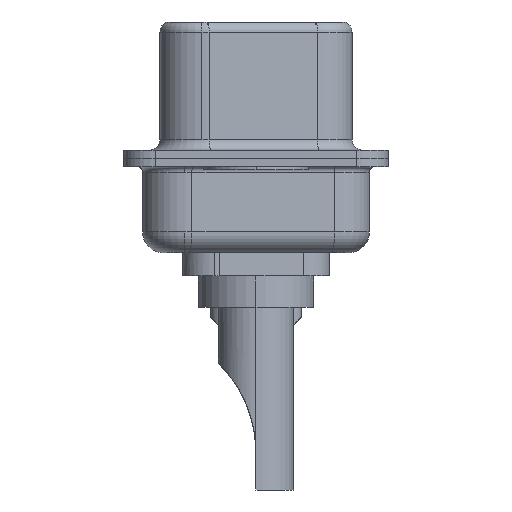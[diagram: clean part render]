
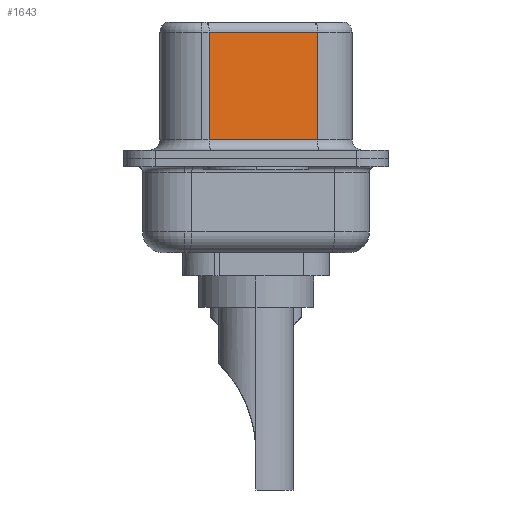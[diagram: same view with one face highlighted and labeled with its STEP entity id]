
A CAD part, left-side view. The second image highlights one B-rep face of the part: STEP entity #1643.
In plain terms, the highlighted planar face has unit normal (-0.985, -0.174, 0).
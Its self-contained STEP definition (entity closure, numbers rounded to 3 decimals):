
#1643 = ADVANCED_FACE ( 'NONE', ( #7416 ), #1813, .F. ) ;
#1660 = EDGE_CURVE ( 'NONE', #17910, #2416, #16244, .T. ) ;
#1813 = PLANE ( 'NONE',  #17124 ) ;
#1856 = CARTESIAN_POINT ( 'NONE',  ( 4.58, -2.927, 6.52 ) ) ;
#2416 = VERTEX_POINT ( 'NONE', #5409 ) ;
#3544 = CARTESIAN_POINT ( 'NONE',  ( 4.58, -2.927, 6.02 ) ) ;
#3776 = VERTEX_POINT ( 'NONE', #17228 ) ;
#3906 = DIRECTION ( 'NONE',  ( -0.174, 0.985, 0. ) ) ;
#4386 = EDGE_CURVE ( 'NONE', #17910, #3776, #13845, .T. ) ;
#4567 = CARTESIAN_POINT ( 'NONE',  ( 4.58, -2.927, 6.02 ) ) ;
#5299 = VECTOR ( 'NONE', #16974, 1000. ) ;
#5409 = CARTESIAN_POINT ( 'NONE',  ( 3.67, 2.233, 6.02 ) ) ;
#5668 = EDGE_CURVE ( 'NONE', #2416, #12429, #13538, .T. ) ;
#6382 = ORIENTED_EDGE ( 'NONE', *, *, #4386, .F. ) ;
#7416 = FACE_OUTER_BOUND ( 'NONE', #19890, .T. ) ;
#9119 = DIRECTION ( 'NONE',  ( 0., 0., -1. ) ) ;
#9835 = LINE ( 'NONE', #10320, #5299 ) ;
#10320 = CARTESIAN_POINT ( 'NONE',  ( 4.58, -2.927, 0.9 ) ) ;
#12429 = VERTEX_POINT ( 'NONE', #21660 ) ;
#13538 = LINE ( 'NONE', #16233, #21734 ) ;
#13790 = ORIENTED_EDGE ( 'NONE', *, *, #1660, .T. ) ;
#13845 = LINE ( 'NONE', #15542, #17678 ) ;
#14345 = ORIENTED_EDGE ( 'NONE', *, *, #5668, .T. ) ;
#15120 = ORIENTED_EDGE ( 'NONE', *, *, #19534, .T. ) ;
#15542 = CARTESIAN_POINT ( 'NONE',  ( 4.58, -2.927, 6.52 ) ) ;
#15750 = VECTOR ( 'NONE', #3906, 1000. ) ;
#16165 = DIRECTION ( 'NONE',  ( 0., 0., -1. ) ) ;
#16233 = CARTESIAN_POINT ( 'NONE',  ( 3.67, 2.233, 6.52 ) ) ;
#16244 = LINE ( 'NONE', #4567, #15750 ) ;
#16762 = DIRECTION ( 'NONE',  ( 0.985, 0.174, 0. ) ) ;
#16974 = DIRECTION ( 'NONE',  ( 0.174, -0.985, 0. ) ) ;
#17124 = AXIS2_PLACEMENT_3D ( 'NONE', #1856, #16762, #17884 ) ;
#17228 = CARTESIAN_POINT ( 'NONE',  ( 4.58, -2.927, 0.9 ) ) ;
#17678 = VECTOR ( 'NONE', #9119, 1000. ) ;
#17884 = DIRECTION ( 'NONE',  ( -0.174, 0.985, 0. ) ) ;
#17910 = VERTEX_POINT ( 'NONE', #3544 ) ;
#19534 = EDGE_CURVE ( 'NONE', #12429, #3776, #9835, .T. ) ;
#19890 = EDGE_LOOP ( 'NONE', ( #6382, #13790, #14345, #15120 ) ) ;
#21660 = CARTESIAN_POINT ( 'NONE',  ( 3.67, 2.233, 0.9 ) ) ;
#21734 = VECTOR ( 'NONE', #16165, 1000. ) ;
